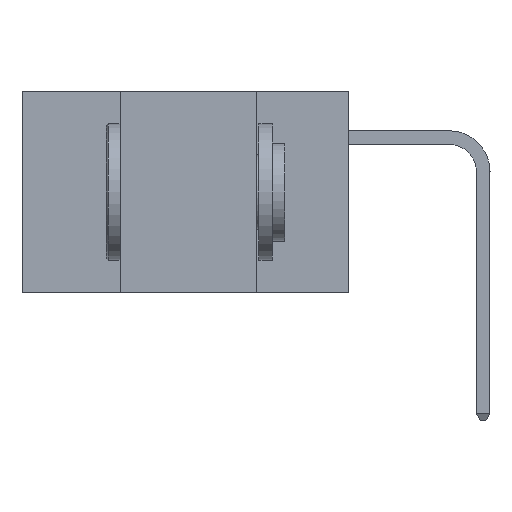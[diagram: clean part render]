
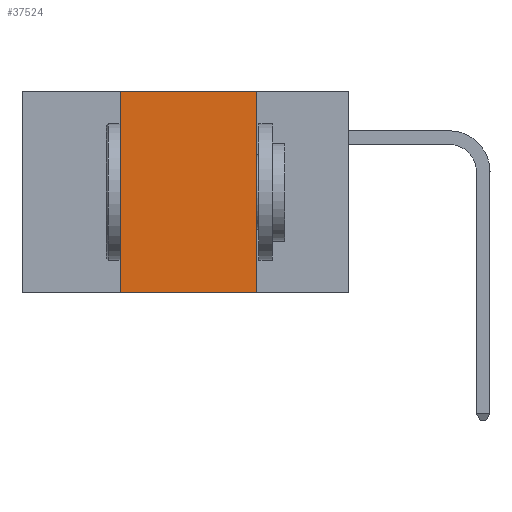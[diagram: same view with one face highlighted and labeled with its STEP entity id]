
A CAD part, left-side view. The second image highlights one B-rep face of the part: STEP entity #37524.
In plain terms, the highlighted planar face has unit normal (-1, 0, 0).
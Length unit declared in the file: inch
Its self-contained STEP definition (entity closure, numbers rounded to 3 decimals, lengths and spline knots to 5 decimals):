
#300 = LINE ( 'NONE', #23261, #15945 ) ;
#2910 = DIRECTION ( 'NONE',  ( 0., 0., -1. ) ) ;
#3011 = DIRECTION ( 'NONE',  ( 0., -1., 0. ) ) ;
#4857 = LINE ( 'NONE', #24734, #36530 ) ;
#5401 = CARTESIAN_POINT ( 'NONE',  ( 0., 0.6, 0. ) ) ;
#6115 = AXIS2_PLACEMENT_3D ( 'NONE', #5401, #39073, #21030 ) ;
#6649 = EDGE_CURVE ( 'NONE', #14209, #18132, #300, .T. ) ;
#6869 = CARTESIAN_POINT ( 'NONE',  ( 0., 0.42, -0.37 ) ) ;
#8575 = FACE_OUTER_BOUND ( 'NONE', #12046, .T. ) ;
#8927 = CARTESIAN_POINT ( 'NONE',  ( 0., 0.17, 0. ) ) ;
#9670 = VECTOR ( 'NONE', #39525, 39.37008 ) ;
#10955 = ORIENTED_EDGE ( 'NONE', *, *, #6649, .F. ) ;
#11918 = ORIENTED_EDGE ( 'NONE', *, *, #36322, .T. ) ;
#12046 = EDGE_LOOP ( 'NONE', ( #30585, #17217, #10955, #11918 ) ) ;
#13712 = LINE ( 'NONE', #24621, #19968 ) ;
#14209 = VERTEX_POINT ( 'NONE', #6869 ) ;
#15945 = VECTOR ( 'NONE', #32313, 39.37008 ) ;
#17217 = ORIENTED_EDGE ( 'NONE', *, *, #33282, .F. ) ;
#17888 = LINE ( 'NONE', #24440, #9670 ) ;
#17941 = PLANE ( 'NONE',  #6115 ) ;
#18132 = VERTEX_POINT ( 'NONE', #36164 ) ;
#19968 = VECTOR ( 'NONE', #2910, 39.37008 ) ;
#21030 = DIRECTION ( 'NONE',  ( 0., 0., -1. ) ) ;
#23261 = CARTESIAN_POINT ( 'NONE',  ( 0., 0.42, 0. ) ) ;
#23862 = VERTEX_POINT ( 'NONE', #39518 ) ;
#24440 = CARTESIAN_POINT ( 'NONE',  ( 0., 0.6, -0.37 ) ) ;
#24621 = CARTESIAN_POINT ( 'NONE',  ( 0., 0.17, 0. ) ) ;
#24734 = CARTESIAN_POINT ( 'NONE',  ( 0., 0.6, 0. ) ) ;
#25809 = VERTEX_POINT ( 'NONE', #8927 ) ;
#28774 = EDGE_CURVE ( 'NONE', #25809, #23862, #13712, .T. ) ;
#30585 = ORIENTED_EDGE ( 'NONE', *, *, #28774, .F. ) ;
#32313 = DIRECTION ( 'NONE',  ( 0., 0., 1. ) ) ;
#33282 = EDGE_CURVE ( 'NONE', #18132, #25809, #4857, .T. ) ;
#36164 = CARTESIAN_POINT ( 'NONE',  ( 0., 0.42, 0. ) ) ;
#36322 = EDGE_CURVE ( 'NONE', #14209, #23862, #17888, .T. ) ;
#36530 = VECTOR ( 'NONE', #3011, 39.37008 ) ;
#37524 = ADVANCED_FACE ( 'NONE', ( #8575 ), #17941, .F. ) ;
#39073 = DIRECTION ( 'NONE',  ( 1., 0., 0. ) ) ;
#39518 = CARTESIAN_POINT ( 'NONE',  ( 0., 0.17, -0.37 ) ) ;
#39525 = DIRECTION ( 'NONE',  ( 0., -1., 0. ) ) ;
